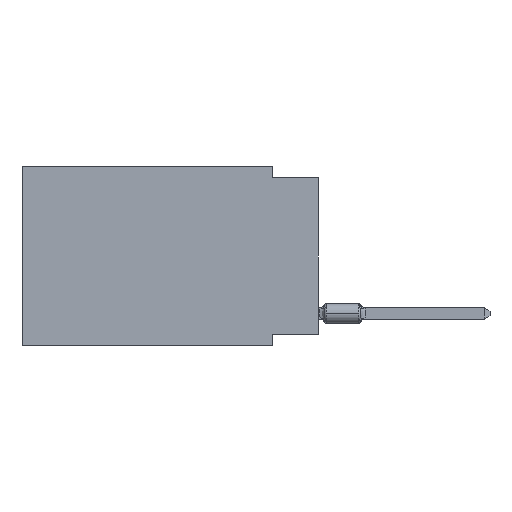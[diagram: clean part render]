
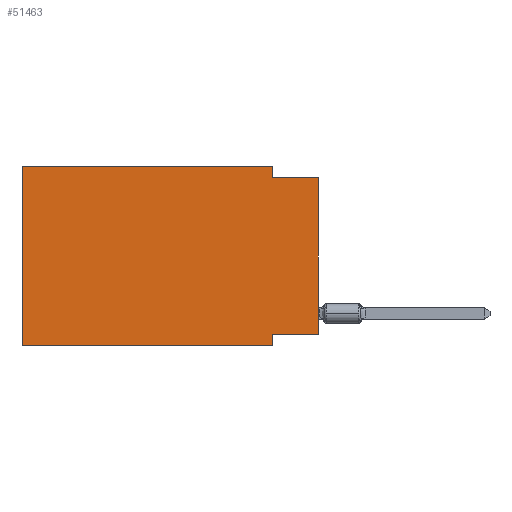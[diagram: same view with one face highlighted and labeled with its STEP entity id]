
A CAD part, left-side view. The second image highlights one B-rep face of the part: STEP entity #51463.
In plain terms, the highlighted planar face has unit normal (-1, 0, 0).
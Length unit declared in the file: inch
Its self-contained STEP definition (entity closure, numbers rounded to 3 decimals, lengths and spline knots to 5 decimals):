
#941 = VERTEX_POINT ( 'NONE', #29395 ) ;
#2399 = ORIENTED_EDGE ( 'NONE', *, *, #43011, .F. ) ;
#2669 = VERTEX_POINT ( 'NONE', #33127 ) ;
#3335 = LINE ( 'NONE', #28781, #43369 ) ;
#3977 = EDGE_CURVE ( 'NONE', #941, #6440, #41459, .T. ) ;
#4276 = EDGE_CURVE ( 'NONE', #57552, #27020, #24354, .T. ) ;
#5300 = CARTESIAN_POINT ( 'NONE',  ( 0., 0.645, 0. ) ) ;
#6440 = VERTEX_POINT ( 'NONE', #60020 ) ;
#7553 = CARTESIAN_POINT ( 'NONE',  ( 0., 0.1, -0.39 ) ) ;
#8152 = LINE ( 'NONE', #49319, #37106 ) ;
#11683 = CARTESIAN_POINT ( 'NONE',  ( 0., 0., 0. ) ) ;
#12450 = VECTOR ( 'NONE', #31686, 39.37008 ) ;
#15494 = DIRECTION ( 'NONE',  ( 1., 0., 0. ) ) ;
#16841 = PLANE ( 'NONE',  #50924 ) ;
#19393 = CARTESIAN_POINT ( 'NONE',  ( 0., 0., -0.365 ) ) ;
#20852 = CARTESIAN_POINT ( 'NONE',  ( 0., 0.645, 0. ) ) ;
#21139 = LINE ( 'NONE', #41866, #28515 ) ;
#22361 = VERTEX_POINT ( 'NONE', #27577 ) ;
#24354 = LINE ( 'NONE', #34059, #44531 ) ;
#26420 = ORIENTED_EDGE ( 'NONE', *, *, #4276, .F. ) ;
#27020 = VERTEX_POINT ( 'NONE', #46535 ) ;
#27577 = CARTESIAN_POINT ( 'NONE',  ( 0., 0.645, -0.39 ) ) ;
#28515 = VECTOR ( 'NONE', #61951, 39.37008 ) ;
#28781 = CARTESIAN_POINT ( 'NONE',  ( 0., 0.1, 0. ) ) ;
#28844 = ORIENTED_EDGE ( 'NONE', *, *, #44049, .F. ) ;
#29120 = ORIENTED_EDGE ( 'NONE', *, *, #44764, .F. ) ;
#29395 = CARTESIAN_POINT ( 'NONE',  ( 0., 0.645, 0. ) ) ;
#31686 = DIRECTION ( 'NONE',  ( 0., -1., 0. ) ) ;
#33127 = CARTESIAN_POINT ( 'NONE',  ( 0., 0., -0.025 ) ) ;
#33702 = VERTEX_POINT ( 'NONE', #38258 ) ;
#34059 = CARTESIAN_POINT ( 'NONE',  ( 0., 0., -0.365 ) ) ;
#34232 = DIRECTION ( 'NONE',  ( 0., -1., 0. ) ) ;
#36557 = CARTESIAN_POINT ( 'NONE',  ( 0., 0.1, -0.025 ) ) ;
#36695 = LINE ( 'NONE', #57131, #12450 ) ;
#37106 = VECTOR ( 'NONE', #34232, 39.37008 ) ;
#38258 = CARTESIAN_POINT ( 'NONE',  ( 0., 0.1, -0.39 ) ) ;
#41459 = LINE ( 'NONE', #5300, #51982 ) ;
#41481 = DIRECTION ( 'NONE',  ( 0., 0., 1. ) ) ;
#41562 = ORIENTED_EDGE ( 'NONE', *, *, #49099, .T. ) ;
#41591 = FACE_OUTER_BOUND ( 'NONE', #52729, .T. ) ;
#41866 = CARTESIAN_POINT ( 'NONE',  ( 0., 0.645, 0. ) ) ;
#42142 = LINE ( 'NONE', #11683, #42283 ) ;
#42283 = VECTOR ( 'NONE', #41481, 39.37008 ) ;
#43011 = EDGE_CURVE ( 'NONE', #6440, #56971, #3335, .T. ) ;
#43369 = VECTOR ( 'NONE', #44527, 39.37008 ) ;
#44049 = EDGE_CURVE ( 'NONE', #22361, #941, #21139, .T. ) ;
#44527 = DIRECTION ( 'NONE',  ( 0., 0., -1. ) ) ;
#44531 = VECTOR ( 'NONE', #59175, 39.37008 ) ;
#44764 = EDGE_CURVE ( 'NONE', #56971, #2669, #8152, .T. ) ;
#45688 = EDGE_CURVE ( 'NONE', #22361, #33702, #36695, .T. ) ;
#46151 = DIRECTION ( 'NONE',  ( 0., -1., 0. ) ) ;
#46535 = CARTESIAN_POINT ( 'NONE',  ( 0., 0.1, -0.365 ) ) ;
#47584 = VECTOR ( 'NONE', #63815, 39.37008 ) ;
#48460 = EDGE_CURVE ( 'NONE', #27020, #33702, #53425, .T. ) ;
#48526 = ORIENTED_EDGE ( 'NONE', *, *, #3977, .F. ) ;
#49099 = EDGE_CURVE ( 'NONE', #57552, #2669, #42142, .T. ) ;
#49319 = CARTESIAN_POINT ( 'NONE',  ( 0., 0., -0.025 ) ) ;
#50609 = ORIENTED_EDGE ( 'NONE', *, *, #48460, .F. ) ;
#50924 = AXIS2_PLACEMENT_3D ( 'NONE', #20852, #15494, #56996 ) ;
#51463 = ADVANCED_FACE ( 'NONE', ( #41591 ), #16841, .F. ) ;
#51982 = VECTOR ( 'NONE', #46151, 39.37008 ) ;
#52729 = EDGE_LOOP ( 'NONE', ( #41562, #29120, #2399, #48526, #28844, #58075, #50609, #26420 ) ) ;
#53425 = LINE ( 'NONE', #7553, #47584 ) ;
#56971 = VERTEX_POINT ( 'NONE', #36557 ) ;
#56996 = DIRECTION ( 'NONE',  ( 0., 0., -1. ) ) ;
#57131 = CARTESIAN_POINT ( 'NONE',  ( 0., 0.645, -0.39 ) ) ;
#57552 = VERTEX_POINT ( 'NONE', #19393 ) ;
#58075 = ORIENTED_EDGE ( 'NONE', *, *, #45688, .T. ) ;
#59175 = DIRECTION ( 'NONE',  ( 0., 1., 0. ) ) ;
#60020 = CARTESIAN_POINT ( 'NONE',  ( 0., 0.1, 0. ) ) ;
#61951 = DIRECTION ( 'NONE',  ( 0., 0., 1. ) ) ;
#63815 = DIRECTION ( 'NONE',  ( 0., 0., -1. ) ) ;
